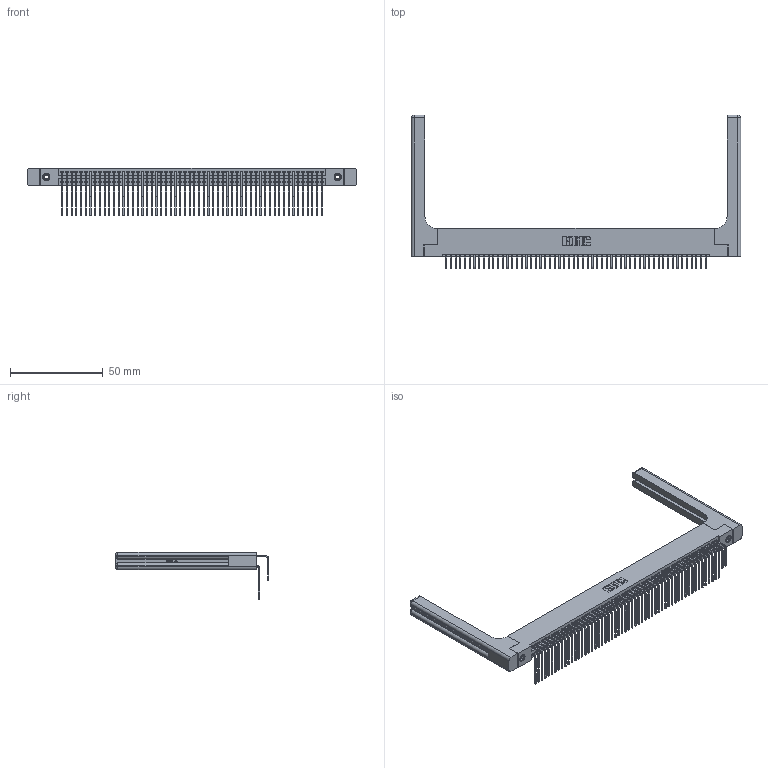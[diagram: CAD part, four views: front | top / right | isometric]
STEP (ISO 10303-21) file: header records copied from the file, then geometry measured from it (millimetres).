
FILE_DESCRIPTION (( 'STEP AP203' ), '1' );
FILE_NAME ('345-112-558-258.STEP', '2019-11-04T23:25:06', ( '' ), ( '' ), 'SwSTEP 2.0', 'SolidWorks 2016', '' );
FILE_SCHEMA (( 'CONFIG_CONTROL_DESIGN' ));
Length unit declared in the file: inch
Products named in the file (6): 345-220-058_345-220-058; 345-292-001_558 559 Tail - 1; 345-112-558-258; 345 Part_Flush Mounting Lugs - 0.156 Dia-TH; 345-292-001_558 Tail - 2; 345-250-001_345-250-001-102
Assembly tree (117 placements, depth 2):
  345-112-558-258
    345 Part_Flush Mounting Lugs - 0.156 Dia-TH
    345-292-001_558 559 Tail - 1  x56
    345-292-001_558 Tail - 2  x56
    345-250-001_345-250-001-102  x2
    345-220-058_345-220-058  x2
Bounding box: 177.27 x 82.79 x 25.53 mm (x, y, z)
Volume: 26471 mm3; surface area: 34969.2 mm2
Topology: 117 solids, 117 shells, 6206 faces, 18367 edges, 12074 vertices
Faces by surface type: plane 4148, cylinder 1998, bspline 36, cone 12, sphere 8, torus 4
Entity records: 48888 total; most frequent: CARTESIAN_POINT 9220, ORIENTED_EDGE 7900, DIRECTION 7018, EDGE_CURVE 3950, VECTOR 3462, LINE 3462, VERTEX_POINT 2622, AXIS2_PLACEMENT_3D 1778
